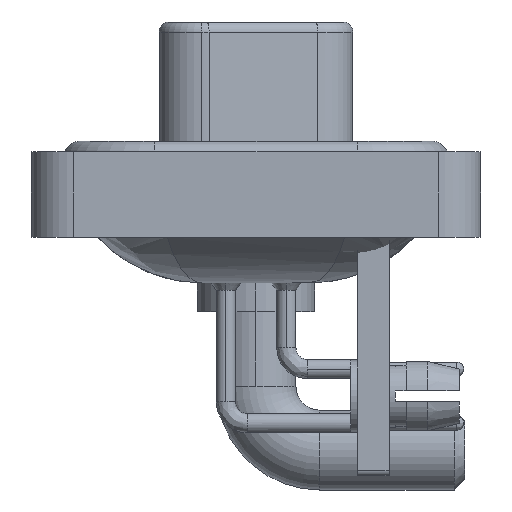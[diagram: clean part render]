
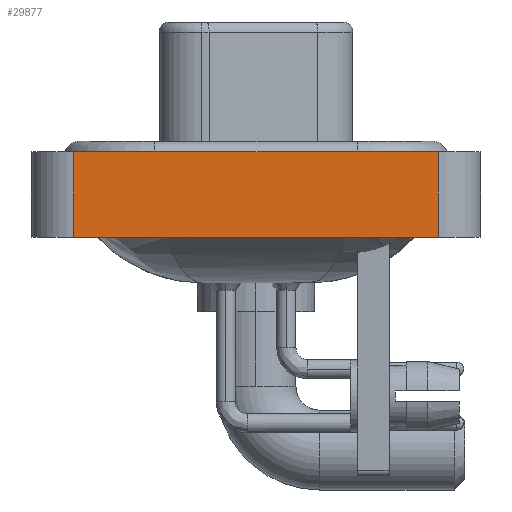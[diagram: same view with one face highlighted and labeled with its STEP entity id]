
A CAD part, left-side view. The second image highlights one B-rep face of the part: STEP entity #29877.
In plain terms, the highlighted planar face has unit normal (-1, 0, 0).
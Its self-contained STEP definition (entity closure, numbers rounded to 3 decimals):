
#1518 = CARTESIAN_POINT ( 'NONE',  ( -7.35, -8.55, -3.6 ) ) ;
#2090 = DIRECTION ( 'NONE',  ( -1., 0., 0. ) ) ;
#2596 = CARTESIAN_POINT ( 'NONE',  ( -7.35, 8.55, 0.4 ) ) ;
#3756 = EDGE_CURVE ( 'NONE', #29962, #14557, #26389, .T. ) ;
#5739 = EDGE_LOOP ( 'NONE', ( #11354, #18752, #9010, #9926 ) ) ;
#5999 = CARTESIAN_POINT ( 'NONE',  ( -7.35, -8.55, 0.4 ) ) ;
#6625 = LINE ( 'NONE', #18452, #8205 ) ;
#8185 = VECTOR ( 'NONE', #25519, 1000. ) ;
#8205 = VECTOR ( 'NONE', #23282, 1000. ) ;
#8268 = DIRECTION ( 'NONE',  ( 0., -1., 0. ) ) ;
#8478 = CARTESIAN_POINT ( 'NONE',  ( -7.35, -8.55, -3.6 ) ) ;
#9010 = ORIENTED_EDGE ( 'NONE', *, *, #13674, .F. ) ;
#9183 = CARTESIAN_POINT ( 'NONE',  ( -7.35, -8.55, 0.4 ) ) ;
#9508 = CARTESIAN_POINT ( 'NONE',  ( -7.35, 8.55, -3.6 ) ) ;
#9926 = ORIENTED_EDGE ( 'NONE', *, *, #3756, .T. ) ;
#10050 = EDGE_CURVE ( 'NONE', #17047, #17811, #30436, .T. ) ;
#10546 = EDGE_CURVE ( 'NONE', #14557, #17811, #15354, .T. ) ;
#10563 = CARTESIAN_POINT ( 'NONE',  ( -7.35, -8.55, -3.6 ) ) ;
#11354 = ORIENTED_EDGE ( 'NONE', *, *, #10546, .T. ) ;
#13674 = EDGE_CURVE ( 'NONE', #29962, #17047, #6625, .T. ) ;
#13771 = DIRECTION ( 'NONE',  ( 0., -1., 0. ) ) ;
#14525 = PLANE ( 'NONE',  #29078 ) ;
#14557 = VERTEX_POINT ( 'NONE', #8478 ) ;
#15354 = LINE ( 'NONE', #25211, #8185 ) ;
#17047 = VERTEX_POINT ( 'NONE', #2596 ) ;
#17811 = VERTEX_POINT ( 'NONE', #9183 ) ;
#18452 = CARTESIAN_POINT ( 'NONE',  ( -7.35, 8.55, -3.6 ) ) ;
#18752 = ORIENTED_EDGE ( 'NONE', *, *, #10050, .F. ) ;
#20234 = VECTOR ( 'NONE', #13771, 1000. ) ;
#23282 = DIRECTION ( 'NONE',  ( 0., 0., 1. ) ) ;
#25122 = FACE_OUTER_BOUND ( 'NONE', #5739, .T. ) ;
#25211 = CARTESIAN_POINT ( 'NONE',  ( -7.35, -8.55, -3.6 ) ) ;
#25289 = DIRECTION ( 'NONE',  ( 0., 0., 1. ) ) ;
#25519 = DIRECTION ( 'NONE',  ( 0., 0., 1. ) ) ;
#26389 = LINE ( 'NONE', #1518, #20234 ) ;
#27821 = VECTOR ( 'NONE', #8268, 1000. ) ;
#29078 = AXIS2_PLACEMENT_3D ( 'NONE', #10563, #2090, #25289 ) ;
#29877 = ADVANCED_FACE ( 'NONE', ( #25122 ), #14525, .T. ) ;
#29962 = VERTEX_POINT ( 'NONE', #9508 ) ;
#30436 = LINE ( 'NONE', #5999, #27821 ) ;
